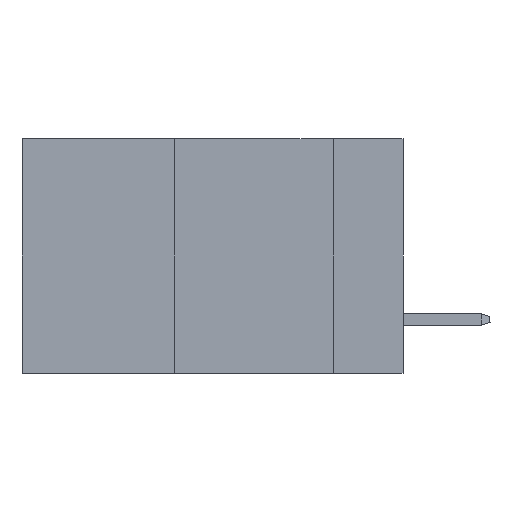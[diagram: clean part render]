
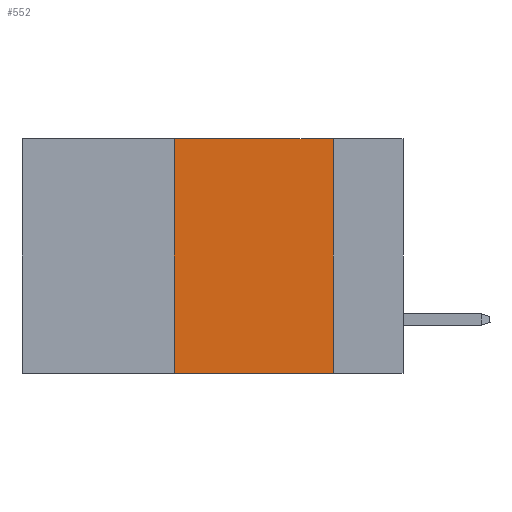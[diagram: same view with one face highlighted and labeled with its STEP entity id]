
A CAD part, left-side view. The second image highlights one B-rep face of the part: STEP entity #552.
In plain terms, the highlighted planar face has unit normal (-1, 0, 0).
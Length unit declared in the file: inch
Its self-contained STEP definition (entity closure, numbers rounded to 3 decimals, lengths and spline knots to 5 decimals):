
#336 = CARTESIAN_POINT ( 'NONE',  ( 0., 0.36, -0.37 ) ) ;
#552 = ADVANCED_FACE ( 'NONE', ( #24815 ), #38091, .F. ) ;
#1324 = VERTEX_POINT ( 'NONE', #40786 ) ;
#1400 = LINE ( 'NONE', #41145, #13817 ) ;
#1714 = AXIS2_PLACEMENT_3D ( 'NONE', #8331, #35667, #41763 ) ;
#4240 = DIRECTION ( 'NONE',  ( 0., 0., 1. ) ) ;
#6478 = DIRECTION ( 'NONE',  ( 0., -1., 0. ) ) ;
#7195 = VERTEX_POINT ( 'NONE', #336 ) ;
#8331 = CARTESIAN_POINT ( 'NONE',  ( 0., 0.6, 0. ) ) ;
#9248 = ORIENTED_EDGE ( 'NONE', *, *, #13734, .F. ) ;
#9926 = VECTOR ( 'NONE', #31820, 39.37008 ) ;
#11958 = VERTEX_POINT ( 'NONE', #20138 ) ;
#12087 = CARTESIAN_POINT ( 'NONE',  ( 0., 0.11, 0. ) ) ;
#12120 = EDGE_CURVE ( 'NONE', #32320, #1324, #18358, .T. ) ;
#13734 = EDGE_CURVE ( 'NONE', #7195, #11958, #1400, .T. ) ;
#13817 = VECTOR ( 'NONE', #4240, 39.37008 ) ;
#14396 = EDGE_LOOP ( 'NONE', ( #17782, #25649, #9248, #20303 ) ) ;
#15206 = CARTESIAN_POINT ( 'NONE',  ( 0., 0.11, 0. ) ) ;
#15384 = CARTESIAN_POINT ( 'NONE',  ( 0., 0.6, -0.37 ) ) ;
#16668 = LINE ( 'NONE', #36218, #29537 ) ;
#17782 = ORIENTED_EDGE ( 'NONE', *, *, #12120, .F. ) ;
#18358 = LINE ( 'NONE', #12087, #9926 ) ;
#18592 = EDGE_CURVE ( 'NONE', #7195, #1324, #32081, .T. ) ;
#18616 = DIRECTION ( 'NONE',  ( 0., -1., 0. ) ) ;
#20138 = CARTESIAN_POINT ( 'NONE',  ( 0., 0.36, 0. ) ) ;
#20303 = ORIENTED_EDGE ( 'NONE', *, *, #18592, .T. ) ;
#24815 = FACE_OUTER_BOUND ( 'NONE', #14396, .T. ) ;
#25649 = ORIENTED_EDGE ( 'NONE', *, *, #27373, .F. ) ;
#27373 = EDGE_CURVE ( 'NONE', #11958, #32320, #16668, .T. ) ;
#27387 = VECTOR ( 'NONE', #18616, 39.37008 ) ;
#29537 = VECTOR ( 'NONE', #6478, 39.37008 ) ;
#31820 = DIRECTION ( 'NONE',  ( 0., 0., -1. ) ) ;
#32081 = LINE ( 'NONE', #15384, #27387 ) ;
#32320 = VERTEX_POINT ( 'NONE', #15206 ) ;
#35667 = DIRECTION ( 'NONE',  ( 1., 0., 0. ) ) ;
#36218 = CARTESIAN_POINT ( 'NONE',  ( 0., 0.6, 0. ) ) ;
#38091 = PLANE ( 'NONE',  #1714 ) ;
#40786 = CARTESIAN_POINT ( 'NONE',  ( 0., 0.11, -0.37 ) ) ;
#41145 = CARTESIAN_POINT ( 'NONE',  ( 0., 0.36, 0. ) ) ;
#41763 = DIRECTION ( 'NONE',  ( 0., 0., -1. ) ) ;
